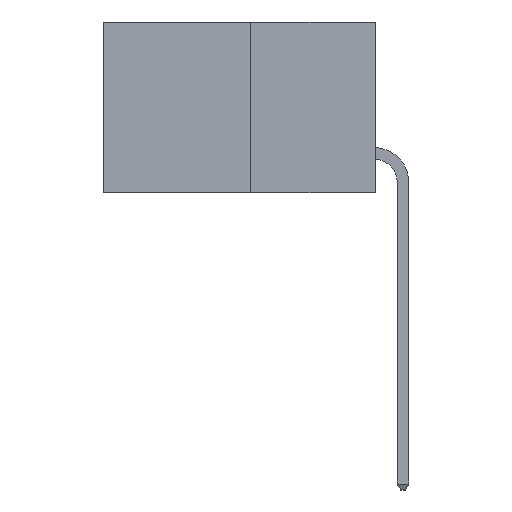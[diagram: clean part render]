
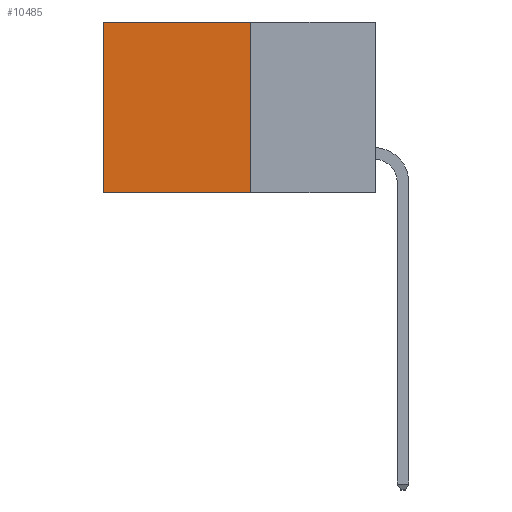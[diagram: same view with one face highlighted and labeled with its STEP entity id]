
A CAD part, left-side view. The second image highlights one B-rep face of the part: STEP entity #10485.
In plain terms, the highlighted planar face has unit normal (-1, 0, 0).
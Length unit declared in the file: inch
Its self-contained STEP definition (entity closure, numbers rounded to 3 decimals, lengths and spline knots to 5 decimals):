
#91 = VERTEX_POINT ( 'NONE', #28914 ) ;
#309 = CARTESIAN_POINT ( 'NONE',  ( 0.277, 0.59, 0. ) ) ;
#2168 = EDGE_CURVE ( 'NONE', #28389, #19077, #18854, .T. ) ;
#3128 = CARTESIAN_POINT ( 'NONE',  ( 0.277, 0.59, -0.37 ) ) ;
#3285 = CARTESIAN_POINT ( 'NONE',  ( 0.277, 0.27, -0.37 ) ) ;
#5398 = LINE ( 'NONE', #3128, #24784 ) ;
#5631 = EDGE_CURVE ( 'NONE', #28133, #91, #26891, .T. ) ;
#5923 = VECTOR ( 'NONE', #13903, 39.37008 ) ;
#7651 = PLANE ( 'NONE',  #22440 ) ;
#7759 = DIRECTION ( 'NONE',  ( 1., 0., 0. ) ) ;
#9163 = EDGE_LOOP ( 'NONE', ( #22957, #19854, #27629, #11536 ) ) ;
#9945 = EDGE_CURVE ( 'NONE', #28389, #28133, #24749, .T. ) ;
#10485 = ADVANCED_FACE ( 'NONE', ( #28086 ), #7651, .F. ) ;
#10665 = DIRECTION ( 'NONE',  ( 0., 0., -1. ) ) ;
#11536 = ORIENTED_EDGE ( 'NONE', *, *, #2168, .T. ) ;
#13136 = CARTESIAN_POINT ( 'NONE',  ( 0.277, 0.27, 0. ) ) ;
#13903 = DIRECTION ( 'NONE',  ( 0., 1., 0. ) ) ;
#17398 = CARTESIAN_POINT ( 'NONE',  ( 0.277, 0.27, -0.37 ) ) ;
#17882 = DIRECTION ( 'NONE',  ( 0., 1., 0. ) ) ;
#18258 = VECTOR ( 'NONE', #10665, 39.37008 ) ;
#18854 = LINE ( 'NONE', #13136, #5923 ) ;
#19077 = VERTEX_POINT ( 'NONE', #309 ) ;
#19854 = ORIENTED_EDGE ( 'NONE', *, *, #5631, .F. ) ;
#22259 = EDGE_CURVE ( 'NONE', #19077, #91, #5398, .T. ) ;
#22440 = AXIS2_PLACEMENT_3D ( 'NONE', #17398, #7759, #24729 ) ;
#22957 = ORIENTED_EDGE ( 'NONE', *, *, #22259, .T. ) ;
#24484 = CARTESIAN_POINT ( 'NONE',  ( 0.277, 0.27, -0.37 ) ) ;
#24729 = DIRECTION ( 'NONE',  ( 0., 0., -1. ) ) ;
#24749 = LINE ( 'NONE', #29909, #18258 ) ;
#24784 = VECTOR ( 'NONE', #25181, 39.37008 ) ;
#25181 = DIRECTION ( 'NONE',  ( 0., 0., -1. ) ) ;
#25362 = VECTOR ( 'NONE', #17882, 39.37008 ) ;
#26891 = LINE ( 'NONE', #3285, #25362 ) ;
#27629 = ORIENTED_EDGE ( 'NONE', *, *, #9945, .F. ) ;
#27721 = CARTESIAN_POINT ( 'NONE',  ( 0.277, 0.27, 0. ) ) ;
#28086 = FACE_OUTER_BOUND ( 'NONE', #9163, .T. ) ;
#28133 = VERTEX_POINT ( 'NONE', #24484 ) ;
#28389 = VERTEX_POINT ( 'NONE', #27721 ) ;
#28914 = CARTESIAN_POINT ( 'NONE',  ( 0.277, 0.59, -0.37 ) ) ;
#29909 = CARTESIAN_POINT ( 'NONE',  ( 0.277, 0.27, -0.37 ) ) ;
